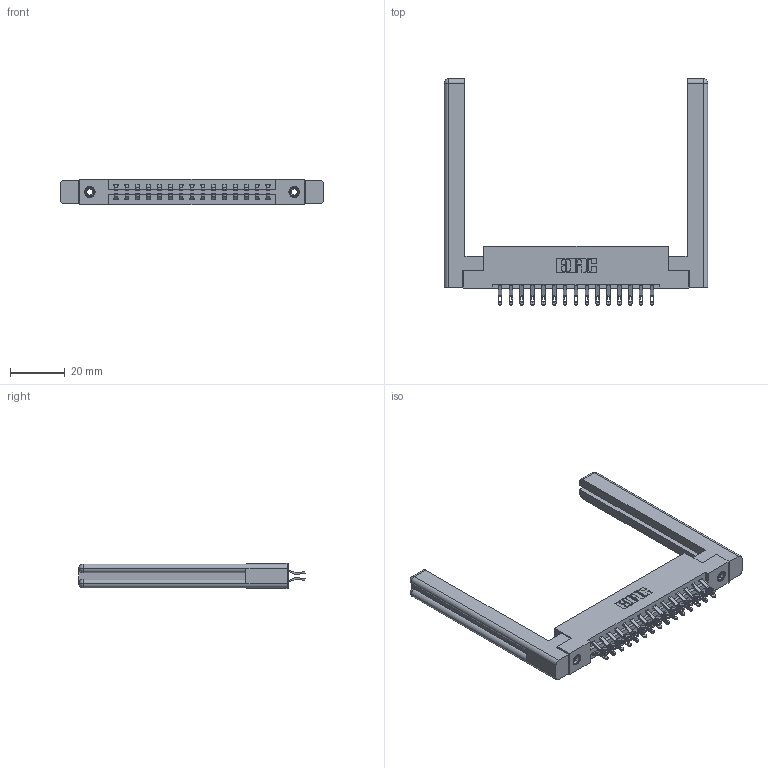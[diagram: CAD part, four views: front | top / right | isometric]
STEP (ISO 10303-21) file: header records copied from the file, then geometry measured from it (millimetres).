
FILE_DESCRIPTION (( 'STEP AP203' ), '1' );
FILE_NAME ('387-030-555-258.STEP', '2019-10-17T14:50:09', ( '' ), ( '' ), 'SwSTEP 2.0', 'SolidWorks 2016', '' );
FILE_SCHEMA (( 'CONFIG_CONTROL_DESIGN' ));
Length unit declared in the file: inch
Products named in the file (5): 307-220-058; 387-030-555-258; 345-250-001_345-250-001-102; 345-292-001_555 Tail; 337 Part_Flush Mounting Lugs - 0.156 Dia-TI
Assembly tree (35 placements, depth 2):
  387-030-555-258
    337 Part_Flush Mounting Lugs - 0.156 Dia-TI
    345-292-001_555 Tail  x30
    345-250-001_345-250-001-102  x2
    307-220-058  x2
Bounding box: 96.06 x 82.56 x 9.4 mm (x, y, z)
Volume: 16993.8 mm3; surface area: 16249.5 mm2
Topology: 35 solids, 35 shells, 2056 faces, 6335 edges, 4210 vertices
Faces by surface type: plane 1234, cylinder 798, cone 12, torus 12
Entity records: 18082 total; most frequent: CARTESIAN_POINT 3111, ORIENTED_EDGE 2956, DIRECTION 2682, EDGE_CURVE 1478, VECTOR 1282, LINE 1282, VERTEX_POINT 978, AXIS2_PLACEMENT_3D 700
